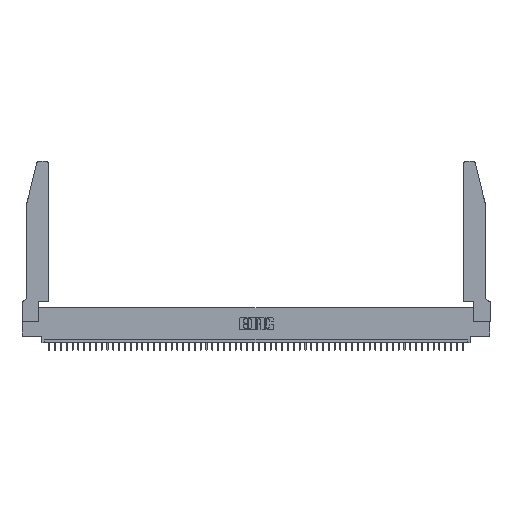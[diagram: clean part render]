
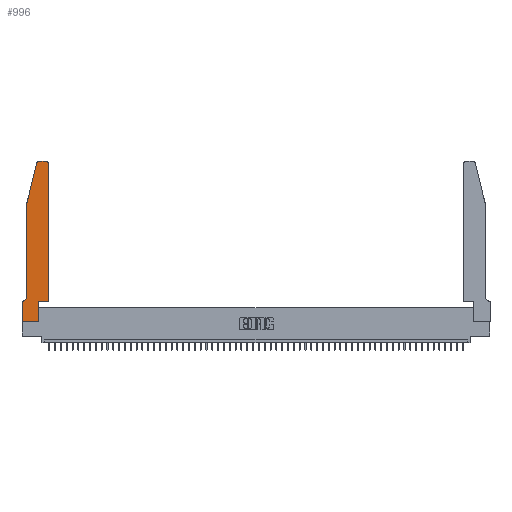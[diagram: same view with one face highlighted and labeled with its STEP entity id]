
A CAD part, top view. The second image highlights one B-rep face of the part: STEP entity #996.
In plain terms, the highlighted planar face has unit normal (0, 0, 1).
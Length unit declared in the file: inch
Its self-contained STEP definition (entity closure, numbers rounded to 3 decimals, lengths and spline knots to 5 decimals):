
#573 = CIRCLE ( 'NONE', #4141, 0.03 ) ;
#615 = EDGE_CURVE ( 'NONE', #44598, #20209, #19894, .T. ) ;
#996 = ADVANCED_FACE ( 'NONE', ( #42689 ), #20921, .T. ) ;
#1505 = VERTEX_POINT ( 'NONE', #33419 ) ;
#1562 = VECTOR ( 'NONE', #11309, 39.37008 ) ;
#2185 = VERTEX_POINT ( 'NONE', #15692 ) ;
#3326 = DIRECTION ( 'NONE',  ( -1., 0., 0. ) ) ;
#3587 = LINE ( 'NONE', #3856, #24830 ) ;
#3856 = CARTESIAN_POINT ( 'NONE',  ( 0.4505, 0.35, 0.37 ) ) ;
#4039 = LINE ( 'NONE', #50887, #29107 ) ;
#4141 = AXIS2_PLACEMENT_3D ( 'NONE', #41081, #31334, #36599 ) ;
#4668 = EDGE_CURVE ( 'NONE', #41065, #16220, #19384, .T. ) ;
#5278 = ORIENTED_EDGE ( 'NONE', *, *, #52017, .T. ) ;
#5737 = CARTESIAN_POINT ( 'NONE',  ( 0., 0.35, 0.37 ) ) ;
#6739 = LINE ( 'NONE', #12597, #9433 ) ;
#6905 = AXIS2_PLACEMENT_3D ( 'NONE', #43708, #22220, #42907 ) ;
#7162 = ORIENTED_EDGE ( 'NONE', *, *, #11742, .T. ) ;
#7492 = ORIENTED_EDGE ( 'NONE', *, *, #27122, .T. ) ;
#8122 = CARTESIAN_POINT ( 'NONE',  ( 0.2865, 0.35, 0.37 ) ) ;
#9044 = VERTEX_POINT ( 'NONE', #26439 ) ;
#9304 = AXIS2_PLACEMENT_3D ( 'NONE', #12290, #47384, #25639 ) ;
#9433 = VECTOR ( 'NONE', #20135, 39.37008 ) ;
#9498 = ORIENTED_EDGE ( 'NONE', *, *, #52152, .T. ) ;
#10832 = VERTEX_POINT ( 'NONE', #21042 ) ;
#11034 = CARTESIAN_POINT ( 'NONE',  ( 0.2865, 0.35, 0.37 ) ) ;
#11309 = DIRECTION ( 'NONE',  ( 0., 1., 0. ) ) ;
#11628 = VECTOR ( 'NONE', #48712, 39.37008 ) ;
#11742 = EDGE_CURVE ( 'NONE', #42451, #9044, #52466, .T. ) ;
#11802 = CARTESIAN_POINT ( 'NONE',  ( 0.0755, 2., 0.37 ) ) ;
#12014 = EDGE_CURVE ( 'NONE', #1505, #2185, #6739, .T. ) ;
#12267 = VERTEX_POINT ( 'NONE', #49061 ) ;
#12290 = CARTESIAN_POINT ( 'NONE',  ( 0., 0.35, 0.37 ) ) ;
#12597 = CARTESIAN_POINT ( 'NONE',  ( 0.4505, 0.35, 0.37 ) ) ;
#14149 = CARTESIAN_POINT ( 'NONE',  ( 0.0755, 0.35, 0.37 ) ) ;
#15240 = ORIENTED_EDGE ( 'NONE', *, *, #45169, .T. ) ;
#15692 = CARTESIAN_POINT ( 'NONE',  ( 0.4505, 2.72, 0.37 ) ) ;
#15896 = DIRECTION ( 'NONE',  ( -1., 0., 0. ) ) ;
#16220 = VERTEX_POINT ( 'NONE', #8122 ) ;
#16421 = DIRECTION ( 'NONE',  ( 1., 0., 0. ) ) ;
#16844 = ORIENTED_EDGE ( 'NONE', *, *, #27270, .T. ) ;
#18630 = LINE ( 'NONE', #14149, #11628 ) ;
#19384 = LINE ( 'NONE', #11034, #1562 ) ;
#19887 = ORIENTED_EDGE ( 'NONE', *, *, #615, .T. ) ;
#19894 = LINE ( 'NONE', #11802, #20892 ) ;
#20135 = DIRECTION ( 'NONE',  ( 0., 1., 0. ) ) ;
#20209 = VERTEX_POINT ( 'NONE', #43035 ) ;
#20614 = ORIENTED_EDGE ( 'NONE', *, *, #12014, .T. ) ;
#20892 = VECTOR ( 'NONE', #53876, 39.37008 ) ;
#20921 = PLANE ( 'NONE',  #9304 ) ;
#21042 = CARTESIAN_POINT ( 'NONE',  ( 0.284, 2.75, 0.37 ) ) ;
#22220 = DIRECTION ( 'NONE',  ( 0., 0., 1. ) ) ;
#24830 = VECTOR ( 'NONE', #16421, 39.37008 ) ;
#25627 = ORIENTED_EDGE ( 'NONE', *, *, #4668, .T. ) ;
#25639 = DIRECTION ( 'NONE',  ( 1., 0., 0. ) ) ;
#26439 = CARTESIAN_POINT ( 'NONE',  ( 0., 0., 0.37 ) ) ;
#27122 = EDGE_CURVE ( 'NONE', #20209, #50491, #4039, .T. ) ;
#27270 = EDGE_CURVE ( 'NONE', #10832, #44598, #573, .T. ) ;
#28180 = DIRECTION ( 'NONE',  ( 0., 0., -1. ) ) ;
#28201 = DIRECTION ( 'NONE',  ( 1., 0., 0. ) ) ;
#29107 = VECTOR ( 'NONE', #29723, 39.37008 ) ;
#29723 = DIRECTION ( 'NONE',  ( 0., -1., 0. ) ) ;
#30240 = EDGE_CURVE ( 'NONE', #2185, #12267, #44349, .T. ) ;
#30562 = VECTOR ( 'NONE', #47489, 39.37008 ) ;
#31334 = DIRECTION ( 'NONE',  ( 0., 0., 1. ) ) ;
#32061 = EDGE_LOOP ( 'NONE', ( #9498, #16844, #19887, #7492, #36041, #40352, #7162, #5278, #25627, #15240, #20614, #38097 ) ) ;
#33419 = CARTESIAN_POINT ( 'NONE',  ( 0.4505, 0.35, 0.37 ) ) ;
#34640 = AXIS2_PLACEMENT_3D ( 'NONE', #45448, #28180, #3326 ) ;
#34925 = CARTESIAN_POINT ( 'NONE',  ( 0., 0., 0.37 ) ) ;
#36041 = ORIENTED_EDGE ( 'NONE', *, *, #45404, .T. ) ;
#36599 = DIRECTION ( 'NONE',  ( 1., 0., 0. ) ) ;
#38097 = ORIENTED_EDGE ( 'NONE', *, *, #30240, .T. ) ;
#38677 = LINE ( 'NONE', #51747, #51051 ) ;
#40352 = ORIENTED_EDGE ( 'NONE', *, *, #46860, .T. ) ;
#41065 = VERTEX_POINT ( 'NONE', #51235 ) ;
#41081 = CARTESIAN_POINT ( 'NONE',  ( 0.284, 2.72, 0.37 ) ) ;
#42451 = VERTEX_POINT ( 'NONE', #5737 ) ;
#42689 = FACE_OUTER_BOUND ( 'NONE', #32061, .T. ) ;
#42718 = CIRCLE ( 'NONE', #34640, 0.07 ) ;
#42907 = DIRECTION ( 'NONE',  ( 1., 0., 0. ) ) ;
#43035 = CARTESIAN_POINT ( 'NONE',  ( 0.0755, 2., 0.37 ) ) ;
#43708 = CARTESIAN_POINT ( 'NONE',  ( 0.4205, 2.72, 0.37 ) ) ;
#44349 = CIRCLE ( 'NONE', #6905, 0.03 ) ;
#44598 = VERTEX_POINT ( 'NONE', #45213 ) ;
#44808 = VECTOR ( 'NONE', #28201, 39.37008 ) ;
#45169 = EDGE_CURVE ( 'NONE', #16220, #1505, #3587, .T. ) ;
#45213 = CARTESIAN_POINT ( 'NONE',  ( 0.25487, 2.72718, 0.37 ) ) ;
#45404 = EDGE_CURVE ( 'NONE', #50491, #53647, #42718, .T. ) ;
#45448 = CARTESIAN_POINT ( 'NONE',  ( 0.0055, 0.42, 0.37 ) ) ;
#45730 = CARTESIAN_POINT ( 'NONE',  ( 0.0755, 0.42, 0.37 ) ) ;
#46860 = EDGE_CURVE ( 'NONE', #53647, #42451, #18630, .T. ) ;
#47384 = DIRECTION ( 'NONE',  ( 0., 0., 1. ) ) ;
#47489 = DIRECTION ( 'NONE',  ( 0., -1., 0. ) ) ;
#48712 = DIRECTION ( 'NONE',  ( -1., 0., 0. ) ) ;
#49061 = CARTESIAN_POINT ( 'NONE',  ( 0.4205, 2.75, 0.37 ) ) ;
#49079 = LINE ( 'NONE', #52694, #44808 ) ;
#50491 = VERTEX_POINT ( 'NONE', #45730 ) ;
#50887 = CARTESIAN_POINT ( 'NONE',  ( 0.0755, 2., 0.37 ) ) ;
#51051 = VECTOR ( 'NONE', #15896, 39.37008 ) ;
#51235 = CARTESIAN_POINT ( 'NONE',  ( 0.2865, 0., 0.37 ) ) ;
#51747 = CARTESIAN_POINT ( 'NONE',  ( 0.2605, 2.75, 0.37 ) ) ;
#52017 = EDGE_CURVE ( 'NONE', #9044, #41065, #49079, .T. ) ;
#52152 = EDGE_CURVE ( 'NONE', #12267, #10832, #38677, .T. ) ;
#52466 = LINE ( 'NONE', #34925, #30562 ) ;
#52694 = CARTESIAN_POINT ( 'NONE',  ( 0., 0., 0.37 ) ) ;
#53159 = CARTESIAN_POINT ( 'NONE',  ( 0.0055, 0.35, 0.37 ) ) ;
#53647 = VERTEX_POINT ( 'NONE', #53159 ) ;
#53876 = DIRECTION ( 'NONE',  ( -0.239, -0.971, 0. ) ) ;
